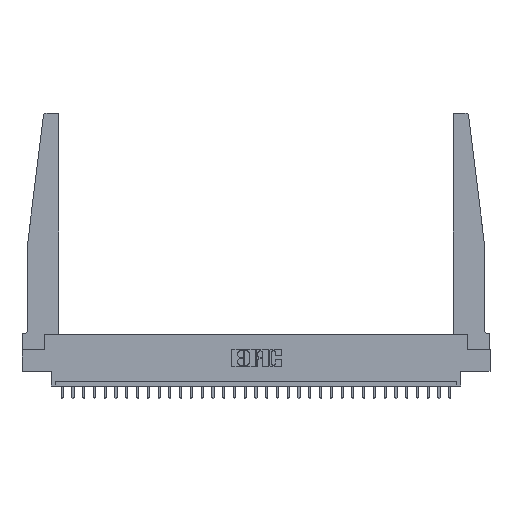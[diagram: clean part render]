
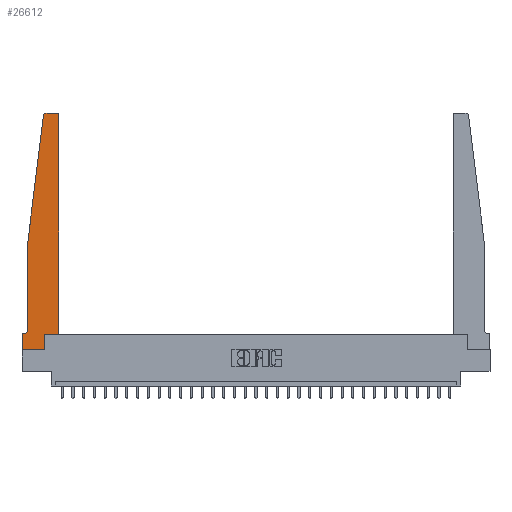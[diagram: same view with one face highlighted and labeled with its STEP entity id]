
A CAD part, top view. The second image highlights one B-rep face of the part: STEP entity #26612.
In plain terms, the highlighted planar face has unit normal (0, 0, 1).
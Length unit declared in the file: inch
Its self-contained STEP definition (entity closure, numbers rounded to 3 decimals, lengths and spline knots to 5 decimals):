
#123 = LINE ( 'NONE', #19940, #10148 ) ;
#901 = CARTESIAN_POINT ( 'NONE',  ( 0., 0., 0.37 ) ) ;
#1117 = CARTESIAN_POINT ( 'NONE',  ( 0.425, 2.72, 0.37 ) ) ;
#1147 = LINE ( 'NONE', #7579, #18014 ) ;
#1522 = LINE ( 'NONE', #23464, #18396 ) ;
#2562 = CARTESIAN_POINT ( 'NONE',  ( 0.27653, 2.75, 0.37 ) ) ;
#2602 = DIRECTION ( 'NONE',  ( 0., 0., 1. ) ) ;
#2778 = VERTEX_POINT ( 'NONE', #16174 ) ;
#3382 = DIRECTION ( 'NONE',  ( 0., 0., 1. ) ) ;
#3851 = CARTESIAN_POINT ( 'NONE',  ( 0.065, 0.2375, 0.37 ) ) ;
#4157 = EDGE_CURVE ( 'NONE', #20259, #7291, #23924, .T. ) ;
#4358 = CARTESIAN_POINT ( 'NONE',  ( 0.25, 2.75, 0.37 ) ) ;
#4628 = CARTESIAN_POINT ( 'NONE',  ( 0.27653, 2.72, 0.37 ) ) ;
#4673 = LINE ( 'NONE', #4358, #15006 ) ;
#4719 = VECTOR ( 'NONE', #21119, 39.37008 ) ;
#4962 = EDGE_CURVE ( 'NONE', #10165, #23802, #20465, .T. ) ;
#5380 = CARTESIAN_POINT ( 'NONE',  ( 0., 0.1875, 0.37 ) ) ;
#5695 = CARTESIAN_POINT ( 'NONE',  ( 0., 0., 0.37 ) ) ;
#7125 = CARTESIAN_POINT ( 'NONE',  ( 0., 0., 0.37 ) ) ;
#7291 = VERTEX_POINT ( 'NONE', #12361 ) ;
#7537 = CARTESIAN_POINT ( 'NONE',  ( 0.395, 2.72, 0.37 ) ) ;
#7579 = CARTESIAN_POINT ( 'NONE',  ( 0.425, 0.18, 0.37 ) ) ;
#7625 = CARTESIAN_POINT ( 'NONE',  ( 0.2605, 0., 0.37 ) ) ;
#8722 = DIRECTION ( 'NONE',  ( 0., 1., 0. ) ) ;
#9058 = DIRECTION ( 'NONE',  ( -0.122, -0.992, 0. ) ) ;
#9074 = DIRECTION ( 'NONE',  ( 1., 0., 0. ) ) ;
#9587 = EDGE_CURVE ( 'NONE', #12857, #11501, #27094, .T. ) ;
#10148 = VECTOR ( 'NONE', #9058, 39.37008 ) ;
#10165 = VERTEX_POINT ( 'NONE', #2562 ) ;
#10223 = DIRECTION ( 'NONE',  ( 0., 0., -1. ) ) ;
#10303 = EDGE_CURVE ( 'NONE', #2778, #10165, #4673, .T. ) ;
#10396 = VERTEX_POINT ( 'NONE', #18802 ) ;
#10416 = DIRECTION ( 'NONE',  ( -1., 0., 0. ) ) ;
#10743 = LINE ( 'NONE', #12890, #21073 ) ;
#10919 = VECTOR ( 'NONE', #27372, 39.37008 ) ;
#10983 = ORIENTED_EDGE ( 'NONE', *, *, #21826, .T. ) ;
#11047 = EDGE_CURVE ( 'NONE', #23802, #10396, #123, .T. ) ;
#11269 = DIRECTION ( 'NONE',  ( 1., 0., 0. ) ) ;
#11495 = DIRECTION ( 'NONE',  ( 0., -1., 0. ) ) ;
#11501 = VERTEX_POINT ( 'NONE', #7625 ) ;
#11944 = CARTESIAN_POINT ( 'NONE',  ( 0.2605, 0.18, 0.37 ) ) ;
#12361 = CARTESIAN_POINT ( 'NONE',  ( 0.015, 0.1875, 0.37 ) ) ;
#12402 = ORIENTED_EDGE ( 'NONE', *, *, #19927, .T. ) ;
#12857 = VERTEX_POINT ( 'NONE', #7125 ) ;
#12890 = CARTESIAN_POINT ( 'NONE',  ( 0.425, 0.18, 0.37 ) ) ;
#13223 = EDGE_LOOP ( 'NONE', ( #21941, #25074, #25478, #23399, #13798, #10983, #12402, #15172, #20299, #14524, #14778, #19374 ) ) ;
#13392 = CARTESIAN_POINT ( 'NONE',  ( 0., 0.1875, 0.37 ) ) ;
#13613 = CARTESIAN_POINT ( 'NONE',  ( 0.065, 1.25, 0.37 ) ) ;
#13798 = ORIENTED_EDGE ( 'NONE', *, *, #4157, .T. ) ;
#14129 = DIRECTION ( 'NONE',  ( 1., 0., 0. ) ) ;
#14274 = LINE ( 'NONE', #11944, #15999 ) ;
#14475 = CARTESIAN_POINT ( 'NONE',  ( 0.015, 0.2375, 0.37 ) ) ;
#14524 = ORIENTED_EDGE ( 'NONE', *, *, #22323, .T. ) ;
#14595 = AXIS2_PLACEMENT_3D ( 'NONE', #14475, #10223, #10416 ) ;
#14778 = ORIENTED_EDGE ( 'NONE', *, *, #25173, .T. ) ;
#14958 = CARTESIAN_POINT ( 'NONE',  ( 0.2605, 0.18, 0.37 ) ) ;
#15006 = VECTOR ( 'NONE', #17766, 39.37008 ) ;
#15172 = ORIENTED_EDGE ( 'NONE', *, *, #9587, .T. ) ;
#15999 = VECTOR ( 'NONE', #16184, 39.37008 ) ;
#16174 = CARTESIAN_POINT ( 'NONE',  ( 0.395, 2.75, 0.37 ) ) ;
#16184 = DIRECTION ( 'NONE',  ( 0., 1., 0. ) ) ;
#16641 = LINE ( 'NONE', #13613, #21793 ) ;
#17077 = CARTESIAN_POINT ( 'NONE',  ( 0.425, 0.18, 0.37 ) ) ;
#17762 = DIRECTION ( 'NONE',  ( 0., 0., 1. ) ) ;
#17766 = DIRECTION ( 'NONE',  ( -1., 0., 0. ) ) ;
#18014 = VECTOR ( 'NONE', #14129, 39.37008 ) ;
#18141 = LINE ( 'NONE', #5695, #4719 ) ;
#18396 = VECTOR ( 'NONE', #25693, 39.37008 ) ;
#18515 = EDGE_CURVE ( 'NONE', #25652, #2778, #25111, .T. ) ;
#18664 = AXIS2_PLACEMENT_3D ( 'NONE', #7537, #3382, #27368 ) ;
#18746 = AXIS2_PLACEMENT_3D ( 'NONE', #13392, #17762, #9074 ) ;
#18802 = CARTESIAN_POINT ( 'NONE',  ( 0.065, 1.25, 0.37 ) ) ;
#19374 = ORIENTED_EDGE ( 'NONE', *, *, #18515, .T. ) ;
#19927 = EDGE_CURVE ( 'NONE', #27352, #12857, #18141, .T. ) ;
#19940 = CARTESIAN_POINT ( 'NONE',  ( 0.065, 1.25, 0.37 ) ) ;
#20259 = VERTEX_POINT ( 'NONE', #3851 ) ;
#20299 = ORIENTED_EDGE ( 'NONE', *, *, #21608, .T. ) ;
#20465 = CIRCLE ( 'NONE', #21411, 0.03 ) ;
#21073 = VECTOR ( 'NONE', #8722, 39.37008 ) ;
#21119 = DIRECTION ( 'NONE',  ( 0., -1., 0. ) ) ;
#21411 = AXIS2_PLACEMENT_3D ( 'NONE', #4628, #2602, #11269 ) ;
#21608 = EDGE_CURVE ( 'NONE', #11501, #25777, #14274, .T. ) ;
#21793 = VECTOR ( 'NONE', #11495, 39.37008 ) ;
#21826 = EDGE_CURVE ( 'NONE', #7291, #27352, #1522, .T. ) ;
#21941 = ORIENTED_EDGE ( 'NONE', *, *, #10303, .T. ) ;
#22179 = CARTESIAN_POINT ( 'NONE',  ( 0.24675, 2.72367, 0.37 ) ) ;
#22323 = EDGE_CURVE ( 'NONE', #25777, #22979, #1147, .T. ) ;
#22979 = VERTEX_POINT ( 'NONE', #17077 ) ;
#23399 = ORIENTED_EDGE ( 'NONE', *, *, #24273, .T. ) ;
#23464 = CARTESIAN_POINT ( 'NONE',  ( 0.065, 0.1875, 0.37 ) ) ;
#23802 = VERTEX_POINT ( 'NONE', #22179 ) ;
#23924 = CIRCLE ( 'NONE', #14595, 0.05 ) ;
#24273 = EDGE_CURVE ( 'NONE', #10396, #20259, #16641, .T. ) ;
#25074 = ORIENTED_EDGE ( 'NONE', *, *, #4962, .T. ) ;
#25111 = CIRCLE ( 'NONE', #18664, 0.03 ) ;
#25173 = EDGE_CURVE ( 'NONE', #22979, #25652, #10743, .T. ) ;
#25447 = FACE_OUTER_BOUND ( 'NONE', #13223, .T. ) ;
#25478 = ORIENTED_EDGE ( 'NONE', *, *, #11047, .T. ) ;
#25652 = VERTEX_POINT ( 'NONE', #1117 ) ;
#25693 = DIRECTION ( 'NONE',  ( -1., 0., 0. ) ) ;
#25777 = VERTEX_POINT ( 'NONE', #14958 ) ;
#26573 = PLANE ( 'NONE',  #18746 ) ;
#26612 = ADVANCED_FACE ( 'NONE', ( #25447 ), #26573, .T. ) ;
#27094 = LINE ( 'NONE', #901, #10919 ) ;
#27352 = VERTEX_POINT ( 'NONE', #5380 ) ;
#27368 = DIRECTION ( 'NONE',  ( 1., 0., 0. ) ) ;
#27372 = DIRECTION ( 'NONE',  ( 1., 0., 0. ) ) ;
